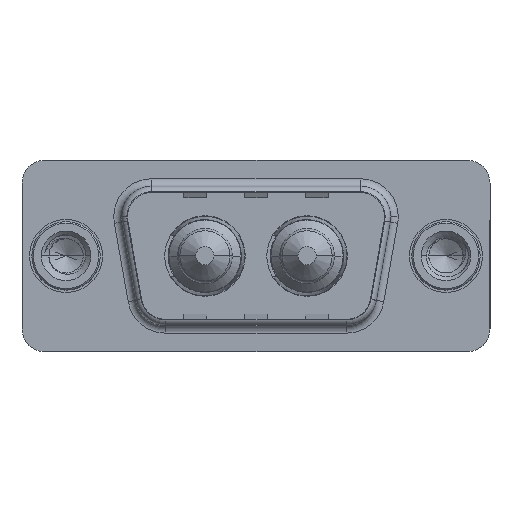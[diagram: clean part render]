
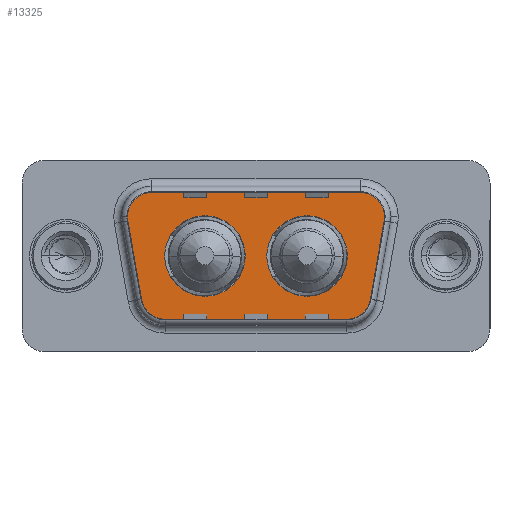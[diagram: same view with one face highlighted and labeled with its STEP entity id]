
A CAD part, top view. The second image highlights one B-rep face of the part: STEP entity #13325.
In plain terms, the highlighted planar face has unit normal (0, 0, 1).
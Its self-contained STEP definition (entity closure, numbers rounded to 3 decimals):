
#7 = DIRECTION ( 'NONE',  ( -1., 0., 0. ) ) ;
#282 = CARTESIAN_POINT ( 'NONE',  ( 18.51, 0., 0. ) ) ;
#325 = EDGE_CURVE ( 'NONE', #11150, #4066, #5553, .T. ) ;
#367 = CIRCLE ( 'NONE', #11781, 2. ) ;
#422 = FACE_BOUND ( 'NONE', #6044, .T. ) ;
#423 = AXIS2_PLACEMENT_3D ( 'NONE', #17229, #8666, #7 ) ;
#776 = DIRECTION ( 'NONE',  ( 0., 0., 1. ) ) ;
#782 = CIRCLE ( 'NONE', #13299, 2. ) ;
#858 = VERTEX_POINT ( 'NONE', #10438 ) ;
#894 = FACE_OUTER_BOUND ( 'NONE', #5821, .T. ) ;
#1105 = DIRECTION ( 'NONE',  ( 0., 0., 1. ) ) ;
#1480 = CARTESIAN_POINT ( 'NONE',  ( 5.436, 4.9, 0. ) ) ;
#1595 = AXIS2_PLACEMENT_3D ( 'NONE', #16271, #10583, #9277 ) ;
#1674 = CARTESIAN_POINT ( 'NONE',  ( 3.466, 2.553, 0. ) ) ;
#1936 = CIRCLE ( 'NONE', #5052, 2.65 ) ;
#2062 = CARTESIAN_POINT ( 'NONE',  ( 4.489, -3.247, 0. ) ) ;
#2115 = AXIS2_PLACEMENT_3D ( 'NONE', #7910, #17916, #9321 ) ;
#2202 = DIRECTION ( 'NONE',  ( 0., 0., 1. ) ) ;
#2223 = ORIENTED_EDGE ( 'NONE', *, *, #3390, .T. ) ;
#2237 = DIRECTION ( 'NONE',  ( 0., 0., 1. ) ) ;
#2306 = VECTOR ( 'NONE', #17605, 1000. ) ;
#2496 = AXIS2_PLACEMENT_3D ( 'NONE', #12537, #1105, #11170 ) ;
#3005 = AXIS2_PLACEMENT_3D ( 'NONE', #10852, #2237, #12276 ) ;
#3390 = EDGE_CURVE ( 'NONE', #4066, #12891, #17545, .T. ) ;
#3585 = CARTESIAN_POINT ( 'NONE',  ( 21.534, 2.553, 0. ) ) ;
#4066 = VERTEX_POINT ( 'NONE', #16701 ) ;
#4210 = EDGE_LOOP ( 'NONE', ( #13657, #17749 ) ) ;
#4237 = CARTESIAN_POINT ( 'NONE',  ( 15.86, 0., 0. ) ) ;
#4269 = FACE_BOUND ( 'NONE', #4210, .T. ) ;
#4641 = LINE ( 'NONE', #9132, #11834 ) ;
#4733 = VECTOR ( 'NONE', #13620, 1000. ) ;
#4734 = VECTOR ( 'NONE', #13477, 1000. ) ;
#4839 = EDGE_CURVE ( 'NONE', #14299, #9050, #12386, .T. ) ;
#5052 = AXIS2_PLACEMENT_3D ( 'NONE', #4237, #14277, #5735 ) ;
#5553 = CIRCLE ( 'NONE', #1595, 2. ) ;
#5612 = ORIENTED_EDGE ( 'NONE', *, *, #15374, .T. ) ;
#5735 = DIRECTION ( 'NONE',  ( 1., 0., 0. ) ) ;
#5779 = VERTEX_POINT ( 'NONE', #13118 ) ;
#5821 = EDGE_LOOP ( 'NONE', ( #15023, #2223, #5612, #12326, #11865, #15232, #14317, #6757, #6308 ) ) ;
#6044 = EDGE_LOOP ( 'NONE', ( #14996, #12119 ) ) ;
#6308 = ORIENTED_EDGE ( 'NONE', *, *, #16711, .T. ) ;
#6578 = VERTEX_POINT ( 'NONE', #9712 ) ;
#6757 = ORIENTED_EDGE ( 'NONE', *, *, #16127, .T. ) ;
#6803 = DIRECTION ( 'NONE',  ( 0., 0., 1. ) ) ;
#7226 = CARTESIAN_POINT ( 'NONE',  ( 13.21, 0., 0. ) ) ;
#7541 = DIRECTION ( 'NONE',  ( 0., 0., 1. ) ) ;
#7845 = EDGE_CURVE ( 'NONE', #6578, #10091, #4641, .T. ) ;
#7910 = CARTESIAN_POINT ( 'NONE',  ( 15.86, 0., 0. ) ) ;
#8666 = DIRECTION ( 'NONE',  ( 0., 0., 1. ) ) ;
#8803 = EDGE_CURVE ( 'NONE', #16523, #9443, #1936, .T. ) ;
#8999 = LINE ( 'NONE', #10764, #4733 ) ;
#9050 = VERTEX_POINT ( 'NONE', #2062 ) ;
#9132 = CARTESIAN_POINT ( 'NONE',  ( 5.436, 4.9, 0. ) ) ;
#9140 = EDGE_CURVE ( 'NONE', #10091, #14299, #782, .T. ) ;
#9277 = DIRECTION ( 'NONE',  ( 1., 0., 0. ) ) ;
#9321 = DIRECTION ( 'NONE',  ( 1., 0., 0. ) ) ;
#9383 = CARTESIAN_POINT ( 'NONE',  ( 5.436, 2.9, 0. ) ) ;
#9443 = VERTEX_POINT ( 'NONE', #7226 ) ;
#9712 = CARTESIAN_POINT ( 'NONE',  ( 19.564, 4.9, 0. ) ) ;
#10091 = VERTEX_POINT ( 'NONE', #1480 ) ;
#10407 = CARTESIAN_POINT ( 'NONE',  ( 18.541, -4.9, 0. ) ) ;
#10438 = CARTESIAN_POINT ( 'NONE',  ( 6.459, -4.9, 0. ) ) ;
#10583 = DIRECTION ( 'NONE',  ( 0., 0., 1. ) ) ;
#10764 = CARTESIAN_POINT ( 'NONE',  ( 6.459, -4.9, 0. ) ) ;
#10809 = CARTESIAN_POINT ( 'NONE',  ( 9.14, 0., 0. ) ) ;
#10848 = DIRECTION ( 'NONE',  ( 1., 0., 0. ) ) ;
#10852 = CARTESIAN_POINT ( 'NONE',  ( 9.14, 0., 0. ) ) ;
#10946 = AXIS2_PLACEMENT_3D ( 'NONE', #16108, #7541, #17525 ) ;
#11150 = VERTEX_POINT ( 'NONE', #10407 ) ;
#11170 = DIRECTION ( 'NONE',  ( 1., 0., 0. ) ) ;
#11781 = AXIS2_PLACEMENT_3D ( 'NONE', #15342, #6803, #16771 ) ;
#11834 = VECTOR ( 'NONE', #12014, 1000. ) ;
#11865 = ORIENTED_EDGE ( 'NONE', *, *, #7845, .T. ) ;
#12014 = DIRECTION ( 'NONE',  ( -1., 0., 0. ) ) ;
#12110 = EDGE_CURVE ( 'NONE', #9443, #16523, #12403, .T. ) ;
#12119 = ORIENTED_EDGE ( 'NONE', *, *, #15595, .F. ) ;
#12236 = DIRECTION ( 'NONE',  ( 1., 0., 0. ) ) ;
#12276 = DIRECTION ( 'NONE',  ( 1., 0., 0. ) ) ;
#12326 = ORIENTED_EDGE ( 'NONE', *, *, #14175, .T. ) ;
#12386 = LINE ( 'NONE', #12487, #4734 ) ;
#12391 = CARTESIAN_POINT ( 'NONE',  ( 21.534, 2.553, 0. ) ) ;
#12403 = CIRCLE ( 'NONE', #2115, 2.65 ) ;
#12487 = CARTESIAN_POINT ( 'NONE',  ( 3.466, 2.553, 0. ) ) ;
#12496 = AXIS2_PLACEMENT_3D ( 'NONE', #10809, #2202, #12236 ) ;
#12537 = CARTESIAN_POINT ( 'NONE',  ( 18.541, -2.9, 0. ) ) ;
#12891 = VERTEX_POINT ( 'NONE', #12391 ) ;
#13118 = CARTESIAN_POINT ( 'NONE',  ( 6.49, 0., 0. ) ) ;
#13299 = AXIS2_PLACEMENT_3D ( 'NONE', #9383, #776, #10848 ) ;
#13325 = ADVANCED_FACE ( 'NONE', ( #4269, #422, #894 ), #16856, .T. ) ;
#13477 = DIRECTION ( 'NONE',  ( 0.174, -0.985, 0. ) ) ;
#13620 = DIRECTION ( 'NONE',  ( 1., 0., 0. ) ) ;
#13657 = ORIENTED_EDGE ( 'NONE', *, *, #8803, .F. ) ;
#13865 = CIRCLE ( 'NONE', #12496, 2.65 ) ;
#14175 = EDGE_CURVE ( 'NONE', #18426, #6578, #16181, .T. ) ;
#14277 = DIRECTION ( 'NONE',  ( 0., 0., 1. ) ) ;
#14299 = VERTEX_POINT ( 'NONE', #1674 ) ;
#14317 = ORIENTED_EDGE ( 'NONE', *, *, #4839, .T. ) ;
#14545 = EDGE_CURVE ( 'NONE', #17277, #5779, #15493, .T. ) ;
#14996 = ORIENTED_EDGE ( 'NONE', *, *, #14545, .F. ) ;
#15023 = ORIENTED_EDGE ( 'NONE', *, *, #325, .T. ) ;
#15232 = ORIENTED_EDGE ( 'NONE', *, *, #9140, .T. ) ;
#15342 = CARTESIAN_POINT ( 'NONE',  ( 6.459, -2.9, 0. ) ) ;
#15374 = EDGE_CURVE ( 'NONE', #12891, #18426, #17022, .T. ) ;
#15493 = CIRCLE ( 'NONE', #3005, 2.65 ) ;
#15595 = EDGE_CURVE ( 'NONE', #5779, #17277, #13865, .T. ) ;
#16108 = CARTESIAN_POINT ( 'NONE',  ( 19.564, 2.9, 0. ) ) ;
#16127 = EDGE_CURVE ( 'NONE', #9050, #858, #367, .T. ) ;
#16181 = CIRCLE ( 'NONE', #423, 2. ) ;
#16271 = CARTESIAN_POINT ( 'NONE',  ( 18.541, -2.9, 0. ) ) ;
#16320 = CARTESIAN_POINT ( 'NONE',  ( 21.564, 2.9, 0. ) ) ;
#16523 = VERTEX_POINT ( 'NONE', #282 ) ;
#16701 = CARTESIAN_POINT ( 'NONE',  ( 20.511, -3.247, 0. ) ) ;
#16711 = EDGE_CURVE ( 'NONE', #858, #11150, #8999, .T. ) ;
#16771 = DIRECTION ( 'NONE',  ( -1., 0., 0. ) ) ;
#16856 = PLANE ( 'NONE',  #2496 ) ;
#17022 = CIRCLE ( 'NONE', #10946, 2. ) ;
#17229 = CARTESIAN_POINT ( 'NONE',  ( 19.564, 2.9, 0. ) ) ;
#17277 = VERTEX_POINT ( 'NONE', #17994 ) ;
#17525 = DIRECTION ( 'NONE',  ( -1., 0., 0. ) ) ;
#17545 = LINE ( 'NONE', #3585, #2306 ) ;
#17605 = DIRECTION ( 'NONE',  ( 0.174, 0.985, 0. ) ) ;
#17749 = ORIENTED_EDGE ( 'NONE', *, *, #12110, .F. ) ;
#17916 = DIRECTION ( 'NONE',  ( 0., 0., 1. ) ) ;
#17994 = CARTESIAN_POINT ( 'NONE',  ( 11.79, 0., 0. ) ) ;
#18426 = VERTEX_POINT ( 'NONE', #16320 ) ;
